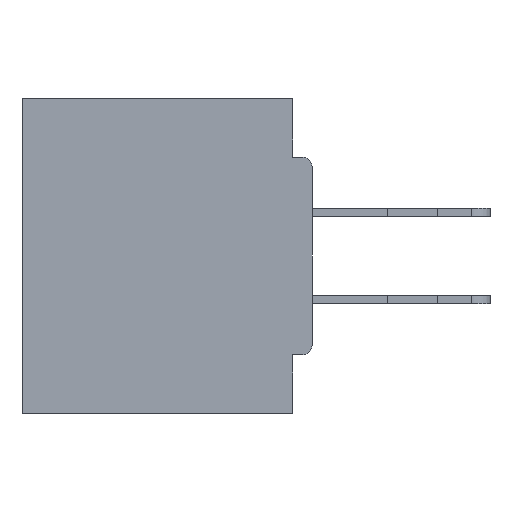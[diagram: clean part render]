
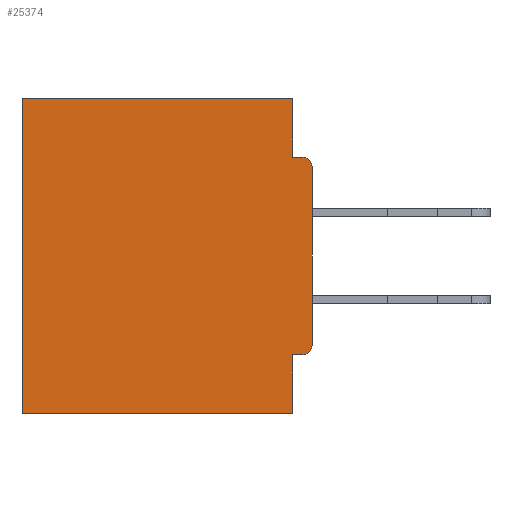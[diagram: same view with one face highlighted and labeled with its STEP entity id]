
A CAD part, left-side view. The second image highlights one B-rep face of the part: STEP entity #25374.
In plain terms, the highlighted planar face has unit normal (-1, 0, 0).
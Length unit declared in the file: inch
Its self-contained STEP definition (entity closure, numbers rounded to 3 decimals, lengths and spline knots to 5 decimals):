
#149 = EDGE_CURVE ( 'NONE', #4805, #10060, #25559, .T. ) ;
#212 = EDGE_LOOP ( 'NONE', ( #22511, #18195, #23277, #37561, #31978, #21426, #6454, #21219, #7762, #12591 ) ) ;
#869 = CARTESIAN_POINT ( 'NONE',  ( 0.298, 0.031, -0.5 ) ) ;
#999 = DIRECTION ( 'NONE',  ( 1., 0., 0. ) ) ;
#2349 = DIRECTION ( 'NONE',  ( 0., -1., 0. ) ) ;
#2507 = VECTOR ( 'NONE', #2349, 39.37008 ) ;
#2769 = EDGE_CURVE ( 'NONE', #14764, #31047, #37427, .T. ) ;
#3296 = VERTEX_POINT ( 'NONE', #869 ) ;
#3770 = VECTOR ( 'NONE', #18198, 39.37008 ) ;
#3827 = VERTEX_POINT ( 'NONE', #14124 ) ;
#4137 = LINE ( 'NONE', #30374, #24542 ) ;
#4254 = EDGE_CURVE ( 'NONE', #14764, #28692, #11925, .T. ) ;
#4805 = VERTEX_POINT ( 'NONE', #6319 ) ;
#5264 = EDGE_CURVE ( 'NONE', #3827, #10060, #34148, .T. ) ;
#5759 = CARTESIAN_POINT ( 'NONE',  ( 0.298, 0.031, -0.5 ) ) ;
#6319 = CARTESIAN_POINT ( 'NONE',  ( 0.298, 0., -0.1085 ) ) ;
#6454 = ORIENTED_EDGE ( 'NONE', *, *, #33498, .F. ) ;
#6786 = EDGE_CURVE ( 'NONE', #20330, #3827, #16784, .T. ) ;
#7762 = ORIENTED_EDGE ( 'NONE', *, *, #2769, .T. ) ;
#8014 = DIRECTION ( 'NONE',  ( 0., 0., -1. ) ) ;
#8571 = CARTESIAN_POINT ( 'NONE',  ( 0.298, 0., -0.0935 ) ) ;
#9092 = CARTESIAN_POINT ( 'NONE',  ( 0.298, 0., 0. ) ) ;
#9314 = LINE ( 'NONE', #25812, #25539 ) ;
#9598 = CARTESIAN_POINT ( 'NONE',  ( 0.298, 0.46, -0.5 ) ) ;
#9661 = CARTESIAN_POINT ( 'NONE',  ( 0.298, 0.015, -0.4065 ) ) ;
#10060 = VERTEX_POINT ( 'NONE', #16516 ) ;
#10286 = LINE ( 'NONE', #12094, #3770 ) ;
#11172 = FACE_OUTER_BOUND ( 'NONE', #212, .T. ) ;
#11686 = DIRECTION ( 'NONE',  ( 0., 0., -1. ) ) ;
#11925 = LINE ( 'NONE', #28316, #16090 ) ;
#12094 = CARTESIAN_POINT ( 'NONE',  ( 0.298, 0., -0.5 ) ) ;
#12591 = ORIENTED_EDGE ( 'NONE', *, *, #30200, .F. ) ;
#13913 = AXIS2_PLACEMENT_3D ( 'NONE', #38286, #999, #37847 ) ;
#14124 = CARTESIAN_POINT ( 'NONE',  ( 0.298, 0.031, -0.0935 ) ) ;
#14764 = VERTEX_POINT ( 'NONE', #9661 ) ;
#14943 = DIRECTION ( 'NONE',  ( -1., 0., 0. ) ) ;
#16090 = VECTOR ( 'NONE', #25042, 39.37008 ) ;
#16516 = CARTESIAN_POINT ( 'NONE',  ( 0.298, 0.015, -0.0935 ) ) ;
#16784 = LINE ( 'NONE', #5759, #23801 ) ;
#16811 = DIRECTION ( 'NONE',  ( 0., 0., -1. ) ) ;
#17458 = PLANE ( 'NONE',  #13913 ) ;
#18195 = ORIENTED_EDGE ( 'NONE', *, *, #5264, .F. ) ;
#18198 = DIRECTION ( 'NONE',  ( 0., 1., 0. ) ) ;
#18853 = LINE ( 'NONE', #23085, #36989 ) ;
#19474 = VERTEX_POINT ( 'NONE', #9598 ) ;
#19607 = EDGE_CURVE ( 'NONE', #20330, #22562, #25841, .T. ) ;
#20325 = DIRECTION ( 'NONE',  ( 0., 0., -1. ) ) ;
#20330 = VERTEX_POINT ( 'NONE', #38264 ) ;
#21219 = ORIENTED_EDGE ( 'NONE', *, *, #4254, .F. ) ;
#21426 = ORIENTED_EDGE ( 'NONE', *, *, #26302, .F. ) ;
#21693 = VECTOR ( 'NONE', #38444, 39.37008 ) ;
#21977 = DIRECTION ( 'NONE',  ( -1., 0., 0. ) ) ;
#22511 = ORIENTED_EDGE ( 'NONE', *, *, #149, .T. ) ;
#22562 = VERTEX_POINT ( 'NONE', #26505 ) ;
#23085 = CARTESIAN_POINT ( 'NONE',  ( 0.298, 0., 0. ) ) ;
#23277 = ORIENTED_EDGE ( 'NONE', *, *, #6786, .F. ) ;
#23517 = DIRECTION ( 'NONE',  ( 0., 0., -1. ) ) ;
#23801 = VECTOR ( 'NONE', #20325, 39.37008 ) ;
#24542 = VECTOR ( 'NONE', #11686, 39.37008 ) ;
#25042 = DIRECTION ( 'NONE',  ( 0., 1., 0. ) ) ;
#25374 = ADVANCED_FACE ( 'NONE', ( #11172 ), #17458, .F. ) ;
#25539 = VECTOR ( 'NONE', #16811, 39.37008 ) ;
#25559 = CIRCLE ( 'NONE', #31454, 0.015 ) ;
#25812 = CARTESIAN_POINT ( 'NONE',  ( 0.298, 0.031, -0.5 ) ) ;
#25841 = LINE ( 'NONE', #9092, #21693 ) ;
#26302 = EDGE_CURVE ( 'NONE', #3296, #19474, #10286, .T. ) ;
#26505 = CARTESIAN_POINT ( 'NONE',  ( 0.298, 0.46, 0. ) ) ;
#27430 = EDGE_CURVE ( 'NONE', #22562, #19474, #4137, .T. ) ;
#28097 = DIRECTION ( 'NONE',  ( 0., 0., -1. ) ) ;
#28316 = CARTESIAN_POINT ( 'NONE',  ( 0.298, 0., -0.4065 ) ) ;
#28692 = VERTEX_POINT ( 'NONE', #34730 ) ;
#29774 = CARTESIAN_POINT ( 'NONE',  ( 0.298, 0.015, -0.3915 ) ) ;
#30200 = EDGE_CURVE ( 'NONE', #4805, #31047, #18853, .T. ) ;
#30374 = CARTESIAN_POINT ( 'NONE',  ( 0.298, 0.46, 0. ) ) ;
#31047 = VERTEX_POINT ( 'NONE', #31631 ) ;
#31454 = AXIS2_PLACEMENT_3D ( 'NONE', #35896, #21977, #28097 ) ;
#31631 = CARTESIAN_POINT ( 'NONE',  ( 0.298, 0., -0.3915 ) ) ;
#31978 = ORIENTED_EDGE ( 'NONE', *, *, #27430, .T. ) ;
#33498 = EDGE_CURVE ( 'NONE', #28692, #3296, #9314, .T. ) ;
#34148 = LINE ( 'NONE', #8571, #2507 ) ;
#34730 = CARTESIAN_POINT ( 'NONE',  ( 0.298, 0.031, -0.4065 ) ) ;
#35896 = CARTESIAN_POINT ( 'NONE',  ( 0.298, 0.015, -0.1085 ) ) ;
#36989 = VECTOR ( 'NONE', #8014, 39.37008 ) ;
#37427 = CIRCLE ( 'NONE', #37481, 0.015 ) ;
#37481 = AXIS2_PLACEMENT_3D ( 'NONE', #29774, #14943, #23517 ) ;
#37561 = ORIENTED_EDGE ( 'NONE', *, *, #19607, .T. ) ;
#37847 = DIRECTION ( 'NONE',  ( 0., 0., -1. ) ) ;
#38264 = CARTESIAN_POINT ( 'NONE',  ( 0.298, 0.031, 0. ) ) ;
#38286 = CARTESIAN_POINT ( 'NONE',  ( 0.298, 0., 0. ) ) ;
#38444 = DIRECTION ( 'NONE',  ( 0., 1., 0. ) ) ;
